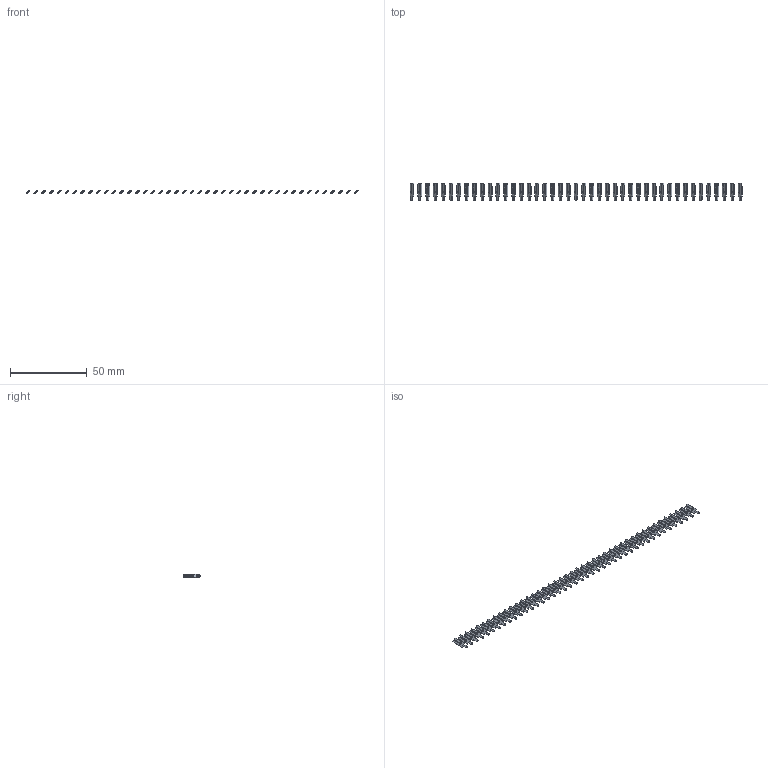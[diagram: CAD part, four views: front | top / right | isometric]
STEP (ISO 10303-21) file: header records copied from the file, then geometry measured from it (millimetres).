
FILE_DESCRIPTION (( 'STEP AP203' ), '1' );
FILE_NAME ('106-043-250-200.STEP', '2020-04-16T20:19:05', ( '' ), ( '' ), 'SwSTEP 2.0', 'SolidWorks 2016', '' );
FILE_SCHEMA (( 'CONFIG_CONTROL_DESIGN' ));
Length unit declared in the file: inch
Products named in the file (2): 106-043-250-200; 100-290-001_100-290-250
Assembly tree (43 placements, depth 2):
  106-043-250-200
    100-290-001_100-290-250  x43
Bounding box: 215.89 x 11.48 x 2.53 mm (x, y, z)
Volume: 671 mm3; surface area: 3154 mm2
Topology: 43 solids, 43 shells, 1032 faces, 2838 edges, 1892 vertices
Faces by surface type: plane 860, cylinder 172
Entity records: 2302 total; most frequent: DIRECTION 210, CARTESIAN_POINT 192, ORIENTED_EDGE 132, COORDINATED_UNIVERSAL_TIME_OFFSET 96, CALENDAR_DATE 96, DATE_AND_TIME 96, LOCAL_TIME 96, AXIS2_PLACEMENT_3D 78
